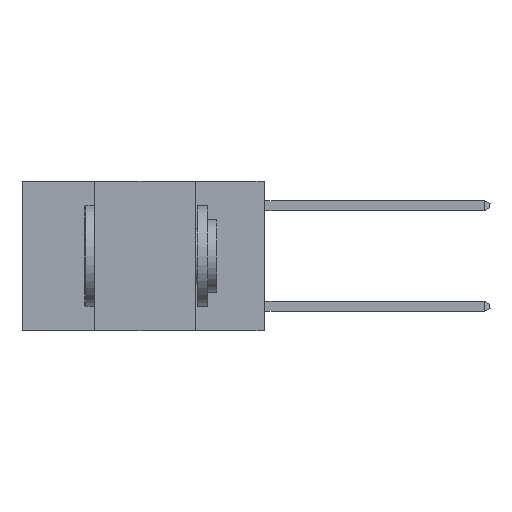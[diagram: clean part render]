
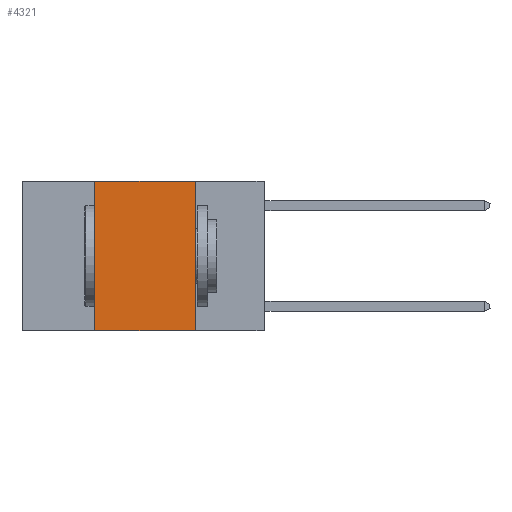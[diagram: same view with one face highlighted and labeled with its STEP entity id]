
A CAD part, left-side view. The second image highlights one B-rep face of the part: STEP entity #4321.
In plain terms, the highlighted planar face has unit normal (-1, 0, 0).
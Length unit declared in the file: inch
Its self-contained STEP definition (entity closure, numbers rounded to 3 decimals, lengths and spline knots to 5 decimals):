
#141 = VECTOR ( 'NONE', #8153, 39.37008 ) ;
#207 = LINE ( 'NONE', #7671, #5776 ) ;
#232 = DIRECTION ( 'NONE',  ( 0., 0., 1. ) ) ;
#339 = ORIENTED_EDGE ( 'NONE', *, *, #11043, .T. ) ;
#507 = VERTEX_POINT ( 'NONE', #919 ) ;
#659 = EDGE_CURVE ( 'NONE', #2162, #5212, #8620, .T. ) ;
#919 = CARTESIAN_POINT ( 'NONE',  ( 0., 0.17, 0. ) ) ;
#1394 = CARTESIAN_POINT ( 'NONE',  ( 0., 0.42, 0. ) ) ;
#1564 = EDGE_CURVE ( 'NONE', #5212, #507, #8212, .T. ) ;
#1756 = VECTOR ( 'NONE', #232, 39.37008 ) ;
#1823 = CARTESIAN_POINT ( 'NONE',  ( 0., 0.42, -0.37 ) ) ;
#2022 = EDGE_CURVE ( 'NONE', #507, #3216, #9099, .T. ) ;
#2162 = VERTEX_POINT ( 'NONE', #1823 ) ;
#2460 = DIRECTION ( 'NONE',  ( 0., 0., -1. ) ) ;
#2511 = DIRECTION ( 'NONE',  ( 1., 0., 0. ) ) ;
#3010 = ORIENTED_EDGE ( 'NONE', *, *, #1564, .F. ) ;
#3216 = VERTEX_POINT ( 'NONE', #7025 ) ;
#3433 = DIRECTION ( 'NONE',  ( 0., 0., -1. ) ) ;
#3576 = CARTESIAN_POINT ( 'NONE',  ( 0., 0.6, 0. ) ) ;
#3783 = ORIENTED_EDGE ( 'NONE', *, *, #659, .F. ) ;
#4321 = ADVANCED_FACE ( 'NONE', ( #8027 ), #5327, .F. ) ;
#5212 = VERTEX_POINT ( 'NONE', #6341 ) ;
#5327 = PLANE ( 'NONE',  #11587 ) ;
#5776 = VECTOR ( 'NONE', #5992, 39.37008 ) ;
#5788 = ORIENTED_EDGE ( 'NONE', *, *, #2022, .F. ) ;
#5992 = DIRECTION ( 'NONE',  ( 0., -1., 0. ) ) ;
#6341 = CARTESIAN_POINT ( 'NONE',  ( 0., 0.42, 0. ) ) ;
#7025 = CARTESIAN_POINT ( 'NONE',  ( 0., 0.17, -0.37 ) ) ;
#7266 = CARTESIAN_POINT ( 'NONE',  ( 0., 0.17, 0. ) ) ;
#7671 = CARTESIAN_POINT ( 'NONE',  ( 0., 0.6, -0.37 ) ) ;
#8027 = FACE_OUTER_BOUND ( 'NONE', #11229, .T. ) ;
#8153 = DIRECTION ( 'NONE',  ( 0., -1., 0. ) ) ;
#8212 = LINE ( 'NONE', #3576, #141 ) ;
#8620 = LINE ( 'NONE', #1394, #1756 ) ;
#9099 = LINE ( 'NONE', #7266, #10805 ) ;
#10805 = VECTOR ( 'NONE', #3433, 39.37008 ) ;
#11043 = EDGE_CURVE ( 'NONE', #2162, #3216, #207, .T. ) ;
#11229 = EDGE_LOOP ( 'NONE', ( #5788, #3010, #3783, #339 ) ) ;
#11587 = AXIS2_PLACEMENT_3D ( 'NONE', #11738, #2511, #2460 ) ;
#11738 = CARTESIAN_POINT ( 'NONE',  ( 0., 0.6, 0. ) ) ;
